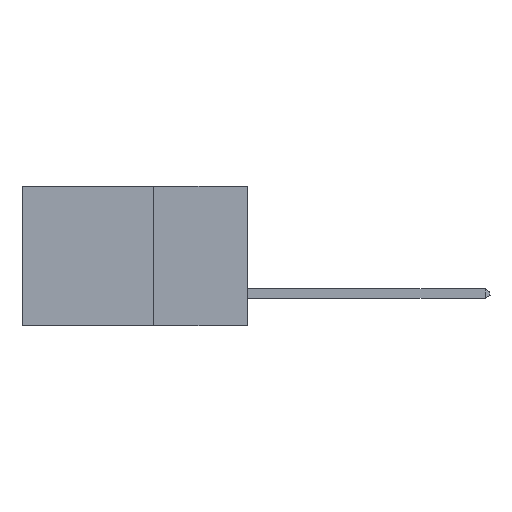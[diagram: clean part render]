
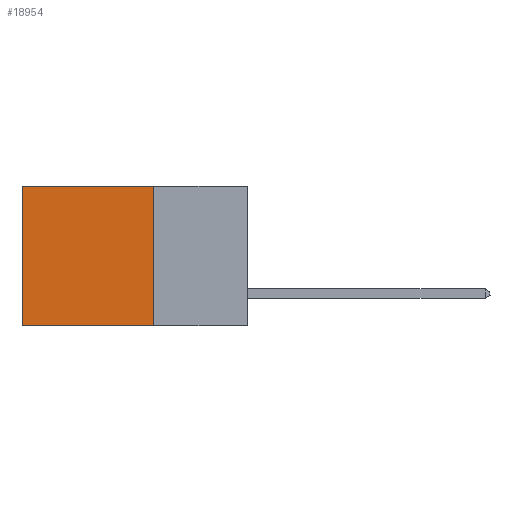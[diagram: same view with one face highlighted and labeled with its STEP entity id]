
A CAD part, left-side view. The second image highlights one B-rep face of the part: STEP entity #18954.
In plain terms, the highlighted planar face has unit normal (-1, 0, 0).
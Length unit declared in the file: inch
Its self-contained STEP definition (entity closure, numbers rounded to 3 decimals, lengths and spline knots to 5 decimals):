
#1533 = VERTEX_POINT ( 'NONE', #18969 ) ;
#1590 = DIRECTION ( 'NONE',  ( 0., 1., 0. ) ) ;
#1956 = EDGE_CURVE ( 'NONE', #19939, #1533, #21364, .T. ) ;
#2073 = CARTESIAN_POINT ( 'NONE',  ( 0.298, 0.6, 0. ) ) ;
#2979 = CARTESIAN_POINT ( 'NONE',  ( 0.298, 0.25, 0. ) ) ;
#3418 = CARTESIAN_POINT ( 'NONE',  ( 0.298, 0.25, 0. ) ) ;
#3429 = ORIENTED_EDGE ( 'NONE', *, *, #9336, .T. ) ;
#3728 = DIRECTION ( 'NONE',  ( 1., 0., 0. ) ) ;
#6685 = VERTEX_POINT ( 'NONE', #18118 ) ;
#7014 = LINE ( 'NONE', #3418, #8195 ) ;
#8003 = CARTESIAN_POINT ( 'NONE',  ( 0.298, 0.25, 0. ) ) ;
#8195 = VECTOR ( 'NONE', #1590, 39.37008 ) ;
#8281 = EDGE_CURVE ( 'NONE', #9566, #19939, #20537, .T. ) ;
#8959 = LINE ( 'NONE', #2073, #17854 ) ;
#9038 = ORIENTED_EDGE ( 'NONE', *, *, #8281, .F. ) ;
#9215 = AXIS2_PLACEMENT_3D ( 'NONE', #12864, #3728, #18567 ) ;
#9336 = EDGE_CURVE ( 'NONE', #6685, #1533, #8959, .T. ) ;
#9566 = VERTEX_POINT ( 'NONE', #2979 ) ;
#9976 = CARTESIAN_POINT ( 'NONE',  ( 0.298, 0.25, -0.37 ) ) ;
#11648 = DIRECTION ( 'NONE',  ( 0., 0., -1. ) ) ;
#12864 = CARTESIAN_POINT ( 'NONE',  ( 0.298, 0.25, 0. ) ) ;
#15216 = VECTOR ( 'NONE', #15723, 39.37008 ) ;
#15637 = DIRECTION ( 'NONE',  ( 0., 0., -1. ) ) ;
#15723 = DIRECTION ( 'NONE',  ( 0., 1., 0. ) ) ;
#16323 = EDGE_CURVE ( 'NONE', #9566, #6685, #7014, .T. ) ;
#17519 = FACE_OUTER_BOUND ( 'NONE', #24462, .T. ) ;
#17854 = VECTOR ( 'NONE', #11648, 39.37008 ) ;
#18118 = CARTESIAN_POINT ( 'NONE',  ( 0.298, 0.6, 0. ) ) ;
#18230 = PLANE ( 'NONE',  #9215 ) ;
#18567 = DIRECTION ( 'NONE',  ( 0., 0., -1. ) ) ;
#18657 = ORIENTED_EDGE ( 'NONE', *, *, #16323, .T. ) ;
#18954 = ADVANCED_FACE ( 'NONE', ( #17519 ), #18230, .F. ) ;
#18969 = CARTESIAN_POINT ( 'NONE',  ( 0.298, 0.6, -0.37 ) ) ;
#19939 = VERTEX_POINT ( 'NONE', #21988 ) ;
#20537 = LINE ( 'NONE', #8003, #21704 ) ;
#21364 = LINE ( 'NONE', #9976, #15216 ) ;
#21704 = VECTOR ( 'NONE', #15637, 39.37008 ) ;
#21988 = CARTESIAN_POINT ( 'NONE',  ( 0.298, 0.25, -0.37 ) ) ;
#24142 = ORIENTED_EDGE ( 'NONE', *, *, #1956, .F. ) ;
#24462 = EDGE_LOOP ( 'NONE', ( #3429, #24142, #9038, #18657 ) ) ;
